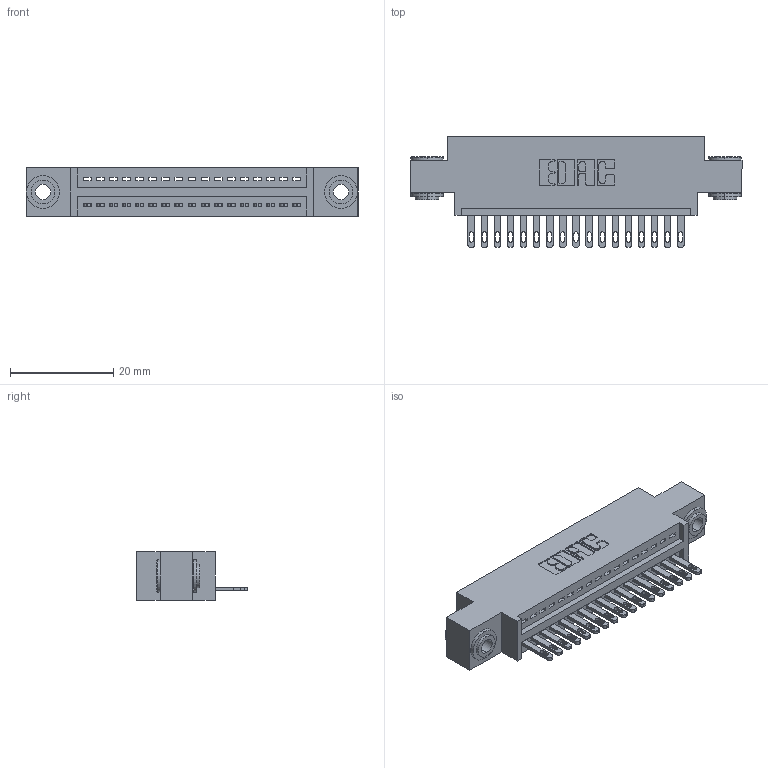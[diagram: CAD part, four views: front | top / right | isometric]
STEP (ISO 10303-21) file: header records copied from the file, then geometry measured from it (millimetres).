
FILE_DESCRIPTION (( 'STEP AP203' ), '1' );
FILE_NAME ('895-017-500-603.STEP', '2020-09-25T05:30:18', ( '' ), ( '' ), 'SwSTEP 2.0', 'SolidWorks 2020', '' );
FILE_SCHEMA (( 'CONFIG_CONTROL_DESIGN' ));
Length unit declared in the file: inch
Products named in the file (4): 895-017-500-603; 345-292-001_345-293-100; 845 Part_0.170 Offset - 0.156 Dia-TH; 345-250-002_345-250-002-102
Assembly tree (20 placements, depth 2):
  895-017-500-603
    845 Part_0.170 Offset - 0.156 Dia-TH
    345-292-001_345-293-100  x17
    345-250-002_345-250-002-102  x2
Bounding box: 64.39 x 21.51 x 9.4 mm (x, y, z)
Volume: 5827.5 mm3; surface area: 7783.6 mm2
Topology: 20 solids, 20 shells, 1086 faces, 3285 edges, 2186 vertices
Faces by surface type: plane 672, cylinder 406, cone 8
Entity records: 16872 total; most frequent: CARTESIAN_POINT 2902, ORIENTED_EDGE 2846, DIRECTION 2603, EDGE_CURVE 1423, LINE 1195, VECTOR 1195, VERTEX_POINT 946, AXIS2_PLACEMENT_3D 704
